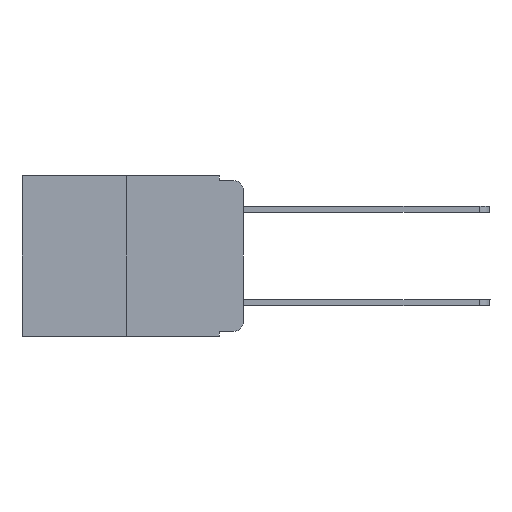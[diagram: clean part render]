
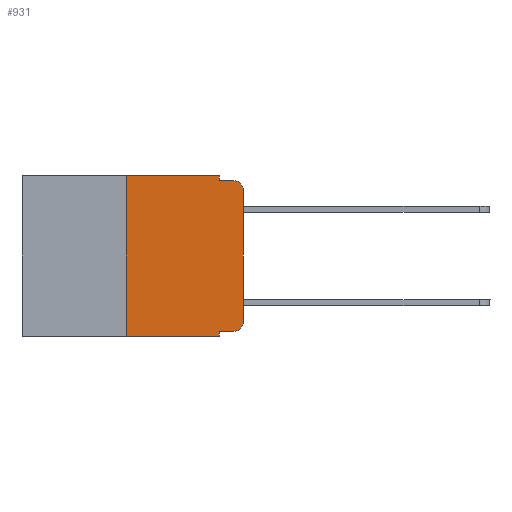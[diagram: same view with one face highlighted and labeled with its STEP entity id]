
A CAD part, left-side view. The second image highlights one B-rep face of the part: STEP entity #931.
In plain terms, the highlighted planar face has unit normal (-1, 0, 0).
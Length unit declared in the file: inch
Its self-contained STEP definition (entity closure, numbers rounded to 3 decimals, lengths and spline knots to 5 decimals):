
#12 = LINE ( 'NONE', #2533, #9372 ) ;
#19 = CARTESIAN_POINT ( 'NONE',  ( 0., 0., -0.03 ) ) ;
#270 = ORIENTED_EDGE ( 'NONE', *, *, #4503, .F. ) ;
#495 = CARTESIAN_POINT ( 'NONE',  ( 0., 0.02, -0.01 ) ) ;
#527 = CARTESIAN_POINT ( 'NONE',  ( 0., 0.051, -0.01 ) ) ;
#607 = VERTEX_POINT ( 'NONE', #495 ) ;
#619 = ORIENTED_EDGE ( 'NONE', *, *, #6574, .T. ) ;
#636 = EDGE_CURVE ( 'NONE', #9945, #5280, #9022, .T. ) ;
#822 = DIRECTION ( 'NONE',  ( 0., 0., -1. ) ) ;
#931 = ADVANCED_FACE ( 'NONE', ( #5978 ), #3269, .F. ) ;
#937 = DIRECTION ( 'NONE',  ( 0., -1., 0. ) ) ;
#1140 = VECTOR ( 'NONE', #6159, 39.37008 ) ;
#1150 = DIRECTION ( 'NONE',  ( 0., -1., 0. ) ) ;
#1408 = EDGE_CURVE ( 'NONE', #6596, #3367, #1464, .T. ) ;
#1433 = LINE ( 'NONE', #4554, #6846 ) ;
#1461 = EDGE_LOOP ( 'NONE', ( #9276, #619, #6287, #270, #2858, #2066, #10815, #7598, #8367, #7810 ) ) ;
#1464 = CIRCLE ( 'NONE', #1471, 0.02 ) ;
#1471 = AXIS2_PLACEMENT_3D ( 'NONE', #5441, #2961, #9703 ) ;
#1640 = DIRECTION ( 'NONE',  ( 0., 0., 1. ) ) ;
#1674 = CARTESIAN_POINT ( 'NONE',  ( 0., 0.051, -0.333 ) ) ;
#1727 = VECTOR ( 'NONE', #1640, 39.37008 ) ;
#1760 = EDGE_CURVE ( 'NONE', #3367, #6747, #10674, .T. ) ;
#1949 = VERTEX_POINT ( 'NONE', #8802 ) ;
#2066 = ORIENTED_EDGE ( 'NONE', *, *, #5959, .F. ) ;
#2518 = CARTESIAN_POINT ( 'NONE',  ( 0., 0.051, 0. ) ) ;
#2533 = CARTESIAN_POINT ( 'NONE',  ( 0., 0.051, 0. ) ) ;
#2557 = CARTESIAN_POINT ( 'NONE',  ( 0., 0.25, 0. ) ) ;
#2605 = CARTESIAN_POINT ( 'NONE',  ( 0., 0.25, -0.343 ) ) ;
#2737 = CARTESIAN_POINT ( 'NONE',  ( 0., 0., 0. ) ) ;
#2858 = ORIENTED_EDGE ( 'NONE', *, *, #636, .F. ) ;
#2961 = DIRECTION ( 'NONE',  ( -1., 0., 0. ) ) ;
#3241 = DIRECTION ( 'NONE',  ( 0., 0., -1. ) ) ;
#3269 = PLANE ( 'NONE',  #9318 ) ;
#3273 = EDGE_CURVE ( 'NONE', #5219, #1949, #10347, .T. ) ;
#3336 = DIRECTION ( 'NONE',  ( 1., 0., 0. ) ) ;
#3367 = VERTEX_POINT ( 'NONE', #9320 ) ;
#3534 = CARTESIAN_POINT ( 'NONE',  ( 0., 0.051, -0.333 ) ) ;
#3634 = AXIS2_PLACEMENT_3D ( 'NONE', #10038, #9935, #8227 ) ;
#4471 = CARTESIAN_POINT ( 'NONE',  ( 0., 0.051, -0.01 ) ) ;
#4503 = EDGE_CURVE ( 'NONE', #5280, #7782, #12, .T. ) ;
#4554 = CARTESIAN_POINT ( 'NONE',  ( 0., 0.473, -0.343 ) ) ;
#4653 = CARTESIAN_POINT ( 'NONE',  ( 0., 0.473, 0. ) ) ;
#5210 = VECTOR ( 'NONE', #7771, 39.37008 ) ;
#5219 = VERTEX_POINT ( 'NONE', #1674 ) ;
#5280 = VERTEX_POINT ( 'NONE', #2518 ) ;
#5431 = EDGE_CURVE ( 'NONE', #7782, #607, #8885, .T. ) ;
#5441 = CARTESIAN_POINT ( 'NONE',  ( 0., 0.02, -0.313 ) ) ;
#5959 = EDGE_CURVE ( 'NONE', #7181, #9945, #9650, .T. ) ;
#5978 = FACE_OUTER_BOUND ( 'NONE', #1461, .T. ) ;
#6159 = DIRECTION ( 'NONE',  ( 0., 0., 1. ) ) ;
#6287 = ORIENTED_EDGE ( 'NONE', *, *, #5431, .F. ) ;
#6364 = CIRCLE ( 'NONE', #3634, 0.02 ) ;
#6574 = EDGE_CURVE ( 'NONE', #6747, #607, #6364, .T. ) ;
#6595 = CARTESIAN_POINT ( 'NONE',  ( 0., 0.051, 0. ) ) ;
#6596 = VERTEX_POINT ( 'NONE', #9167 ) ;
#6747 = VERTEX_POINT ( 'NONE', #19 ) ;
#6846 = VECTOR ( 'NONE', #8745, 39.37008 ) ;
#6863 = CARTESIAN_POINT ( 'NONE',  ( 0., 0.25, 0. ) ) ;
#7181 = VERTEX_POINT ( 'NONE', #2605 ) ;
#7184 = VECTOR ( 'NONE', #1150, 39.37008 ) ;
#7366 = EDGE_CURVE ( 'NONE', #7181, #1949, #1433, .T. ) ;
#7598 = ORIENTED_EDGE ( 'NONE', *, *, #3273, .F. ) ;
#7619 = CARTESIAN_POINT ( 'NONE',  ( 0., 0.473, 0. ) ) ;
#7771 = DIRECTION ( 'NONE',  ( 0., -1., 0. ) ) ;
#7782 = VERTEX_POINT ( 'NONE', #527 ) ;
#7810 = ORIENTED_EDGE ( 'NONE', *, *, #1408, .T. ) ;
#8101 = VECTOR ( 'NONE', #3241, 39.37008 ) ;
#8227 = DIRECTION ( 'NONE',  ( 0., 0., -1. ) ) ;
#8339 = VECTOR ( 'NONE', #937, 39.37008 ) ;
#8367 = ORIENTED_EDGE ( 'NONE', *, *, #9374, .T. ) ;
#8745 = DIRECTION ( 'NONE',  ( 0., -1., 0. ) ) ;
#8802 = CARTESIAN_POINT ( 'NONE',  ( 0., 0.051, -0.343 ) ) ;
#8885 = LINE ( 'NONE', #4471, #8339 ) ;
#9022 = LINE ( 'NONE', #4653, #5210 ) ;
#9167 = CARTESIAN_POINT ( 'NONE',  ( 0., 0.02, -0.333 ) ) ;
#9276 = ORIENTED_EDGE ( 'NONE', *, *, #1760, .T. ) ;
#9281 = LINE ( 'NONE', #3534, #7184 ) ;
#9318 = AXIS2_PLACEMENT_3D ( 'NONE', #7619, #3336, #822 ) ;
#9320 = CARTESIAN_POINT ( 'NONE',  ( 0., 0., -0.313 ) ) ;
#9372 = VECTOR ( 'NONE', #10026, 39.37008 ) ;
#9374 = EDGE_CURVE ( 'NONE', #5219, #6596, #9281, .T. ) ;
#9650 = LINE ( 'NONE', #2557, #1727 ) ;
#9703 = DIRECTION ( 'NONE',  ( 0., 0., -1. ) ) ;
#9935 = DIRECTION ( 'NONE',  ( -1., 0., 0. ) ) ;
#9945 = VERTEX_POINT ( 'NONE', #6863 ) ;
#10026 = DIRECTION ( 'NONE',  ( 0., 0., -1. ) ) ;
#10038 = CARTESIAN_POINT ( 'NONE',  ( 0., 0.02, -0.03 ) ) ;
#10347 = LINE ( 'NONE', #6595, #8101 ) ;
#10674 = LINE ( 'NONE', #2737, #1140 ) ;
#10815 = ORIENTED_EDGE ( 'NONE', *, *, #7366, .T. ) ;
